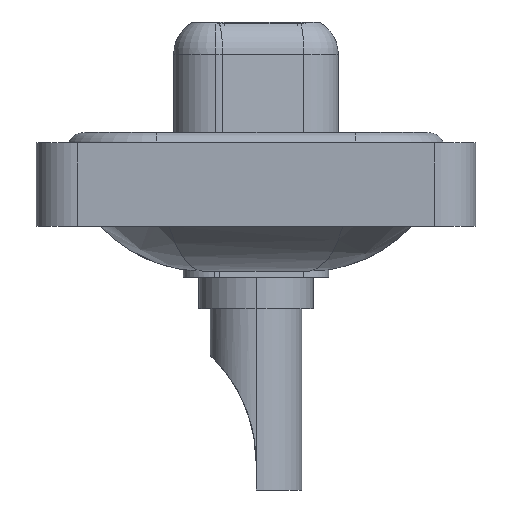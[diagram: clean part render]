
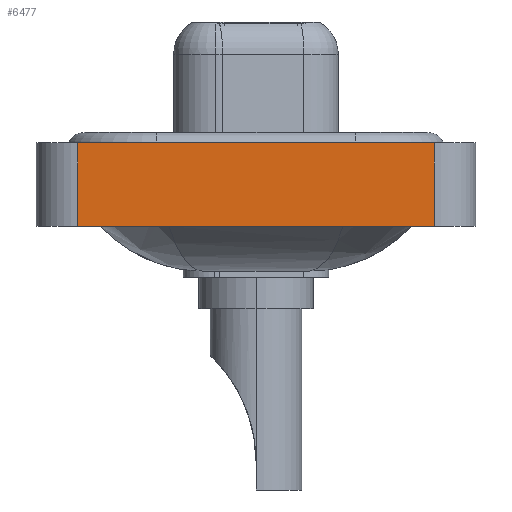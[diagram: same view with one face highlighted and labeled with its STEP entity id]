
A CAD part, left-side view. The second image highlights one B-rep face of the part: STEP entity #6477.
In plain terms, the highlighted planar face has unit normal (-1, 0, 0).
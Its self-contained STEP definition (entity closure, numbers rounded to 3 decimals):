
#210 = VERTEX_POINT ( 'NONE', #13041 ) ;
#318 = FACE_OUTER_BOUND ( 'NONE', #10491, .T. ) ;
#902 = ORIENTED_EDGE ( 'NONE', *, *, #8917, .T. ) ;
#971 = EDGE_CURVE ( 'NONE', #210, #8507, #5498, .T. ) ;
#1470 = ORIENTED_EDGE ( 'NONE', *, *, #15317, .F. ) ;
#1695 = CARTESIAN_POINT ( 'NONE',  ( -7.25, -8.55, -3.6 ) ) ;
#4065 = DIRECTION ( 'NONE',  ( 0., 0., 1. ) ) ;
#5203 = DIRECTION ( 'NONE',  ( 0., 0., 1. ) ) ;
#5246 = EDGE_CURVE ( 'NONE', #5502, #8507, #9488, .T. ) ;
#5498 = LINE ( 'NONE', #11326, #15453 ) ;
#5502 = VERTEX_POINT ( 'NONE', #9082 ) ;
#6065 = CARTESIAN_POINT ( 'NONE',  ( -7.25, -8.55, 0.4 ) ) ;
#6477 = ADVANCED_FACE ( 'NONE', ( #318 ), #13852, .T. ) ;
#7007 = CARTESIAN_POINT ( 'NONE',  ( -7.25, -8.55, 0.4 ) ) ;
#7152 = AXIS2_PLACEMENT_3D ( 'NONE', #1695, #10086, #5203 ) ;
#7161 = VERTEX_POINT ( 'NONE', #15281 ) ;
#7207 = VECTOR ( 'NONE', #8648, 1000. ) ;
#8049 = ORIENTED_EDGE ( 'NONE', *, *, #971, .T. ) ;
#8507 = VERTEX_POINT ( 'NONE', #6065 ) ;
#8519 = CARTESIAN_POINT ( 'NONE',  ( -7.25, -8.55, -3.6 ) ) ;
#8648 = DIRECTION ( 'NONE',  ( 0., 0., 1. ) ) ;
#8917 = EDGE_CURVE ( 'NONE', #7161, #210, #15818, .T. ) ;
#9082 = CARTESIAN_POINT ( 'NONE',  ( -7.25, 8.55, 0.4 ) ) ;
#9488 = LINE ( 'NONE', #7007, #9874 ) ;
#9874 = VECTOR ( 'NONE', #14296, 1000. ) ;
#10086 = DIRECTION ( 'NONE',  ( -1., 0., 0. ) ) ;
#10491 = EDGE_LOOP ( 'NONE', ( #8049, #13741, #1470, #902 ) ) ;
#11044 = LINE ( 'NONE', #12251, #7207 ) ;
#11117 = VECTOR ( 'NONE', #13423, 1000. ) ;
#11326 = CARTESIAN_POINT ( 'NONE',  ( -7.25, -8.55, -3.6 ) ) ;
#12251 = CARTESIAN_POINT ( 'NONE',  ( -7.25, 8.55, -3.6 ) ) ;
#13041 = CARTESIAN_POINT ( 'NONE',  ( -7.25, -8.55, -3.6 ) ) ;
#13423 = DIRECTION ( 'NONE',  ( 0., -1., 0. ) ) ;
#13741 = ORIENTED_EDGE ( 'NONE', *, *, #5246, .F. ) ;
#13852 = PLANE ( 'NONE',  #7152 ) ;
#14296 = DIRECTION ( 'NONE',  ( 0., -1., 0. ) ) ;
#15281 = CARTESIAN_POINT ( 'NONE',  ( -7.25, 8.55, -3.6 ) ) ;
#15317 = EDGE_CURVE ( 'NONE', #7161, #5502, #11044, .T. ) ;
#15453 = VECTOR ( 'NONE', #4065, 1000. ) ;
#15818 = LINE ( 'NONE', #8519, #11117 ) ;
